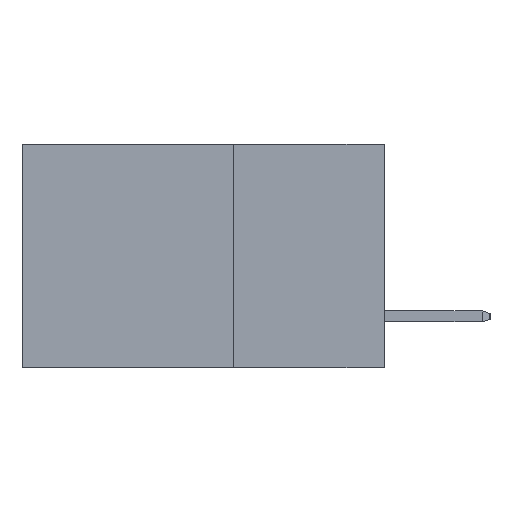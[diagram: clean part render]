
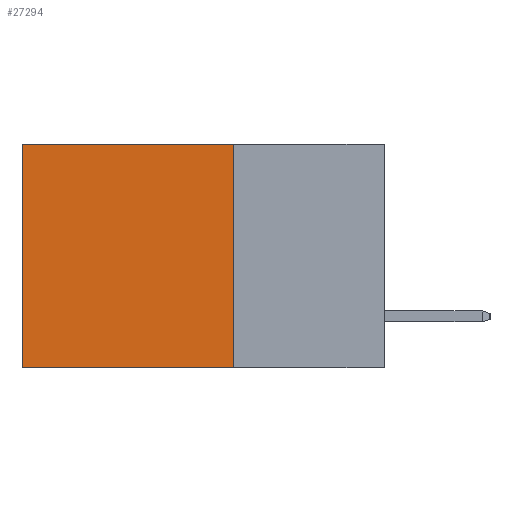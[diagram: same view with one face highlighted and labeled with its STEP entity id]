
A CAD part, left-side view. The second image highlights one B-rep face of the part: STEP entity #27294.
In plain terms, the highlighted planar face has unit normal (-1, 0, 0).
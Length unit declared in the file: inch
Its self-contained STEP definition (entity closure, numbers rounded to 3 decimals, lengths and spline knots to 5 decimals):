
#675 = EDGE_CURVE ( 'NONE', #12009, #24620, #23946, .T. ) ;
#2465 = CARTESIAN_POINT ( 'NONE',  ( 0.298, 0.25, -0.37 ) ) ;
#2511 = VECTOR ( 'NONE', #10066, 39.37008 ) ;
#4812 = DIRECTION ( 'NONE',  ( 0., 1., 0. ) ) ;
#5656 = CARTESIAN_POINT ( 'NONE',  ( 0.298, 0.25, 0. ) ) ;
#5689 = ORIENTED_EDGE ( 'NONE', *, *, #7837, .F. ) ;
#6432 = PLANE ( 'NONE',  #16565 ) ;
#7837 = EDGE_CURVE ( 'NONE', #9963, #18147, #8273, .T. ) ;
#8229 = ORIENTED_EDGE ( 'NONE', *, *, #9858, .T. ) ;
#8273 = LINE ( 'NONE', #5656, #2511 ) ;
#8313 = CARTESIAN_POINT ( 'NONE',  ( 0.298, 0.25, -0.37 ) ) ;
#8991 = DIRECTION ( 'NONE',  ( 0., 1., 0. ) ) ;
#9513 = CARTESIAN_POINT ( 'NONE',  ( 0.298, 0.6, -0.37 ) ) ;
#9858 = EDGE_CURVE ( 'NONE', #9963, #12009, #20874, .T. ) ;
#9963 = VERTEX_POINT ( 'NONE', #14220 ) ;
#10066 = DIRECTION ( 'NONE',  ( 0., 0., -1. ) ) ;
#10452 = EDGE_LOOP ( 'NONE', ( #23308, #23158, #5689, #8229 ) ) ;
#11614 = VECTOR ( 'NONE', #8991, 39.37008 ) ;
#12009 = VERTEX_POINT ( 'NONE', #22699 ) ;
#14220 = CARTESIAN_POINT ( 'NONE',  ( 0.298, 0.25, 0. ) ) ;
#15303 = VECTOR ( 'NONE', #4812, 39.37008 ) ;
#16565 = AXIS2_PLACEMENT_3D ( 'NONE', #17196, #19196, #21371 ) ;
#16690 = CARTESIAN_POINT ( 'NONE',  ( 0.298, 0.6, 0. ) ) ;
#16967 = DIRECTION ( 'NONE',  ( 0., 0., -1. ) ) ;
#17196 = CARTESIAN_POINT ( 'NONE',  ( 0.298, 0.25, 0. ) ) ;
#17251 = LINE ( 'NONE', #2465, #11614 ) ;
#17797 = VECTOR ( 'NONE', #16967, 39.37008 ) ;
#18147 = VERTEX_POINT ( 'NONE', #8313 ) ;
#19196 = DIRECTION ( 'NONE',  ( 1., 0., 0. ) ) ;
#19913 = FACE_OUTER_BOUND ( 'NONE', #10452, .T. ) ;
#20130 = EDGE_CURVE ( 'NONE', #18147, #24620, #17251, .T. ) ;
#20874 = LINE ( 'NONE', #26002, #15303 ) ;
#21371 = DIRECTION ( 'NONE',  ( 0., 0., -1. ) ) ;
#22699 = CARTESIAN_POINT ( 'NONE',  ( 0.298, 0.6, 0. ) ) ;
#23158 = ORIENTED_EDGE ( 'NONE', *, *, #20130, .F. ) ;
#23308 = ORIENTED_EDGE ( 'NONE', *, *, #675, .T. ) ;
#23946 = LINE ( 'NONE', #16690, #17797 ) ;
#24620 = VERTEX_POINT ( 'NONE', #9513 ) ;
#26002 = CARTESIAN_POINT ( 'NONE',  ( 0.298, 0.25, 0. ) ) ;
#27294 = ADVANCED_FACE ( 'NONE', ( #19913 ), #6432, .F. ) ;
